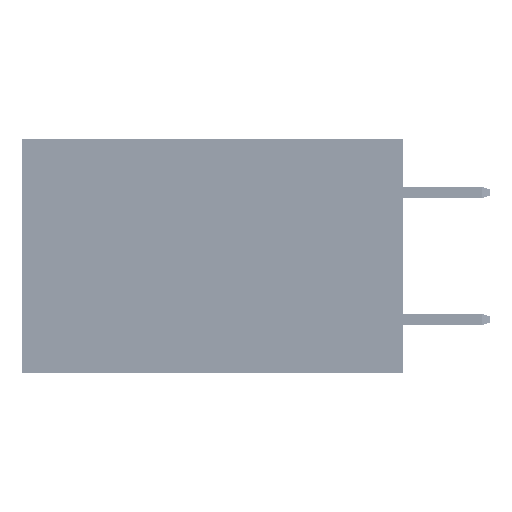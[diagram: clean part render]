
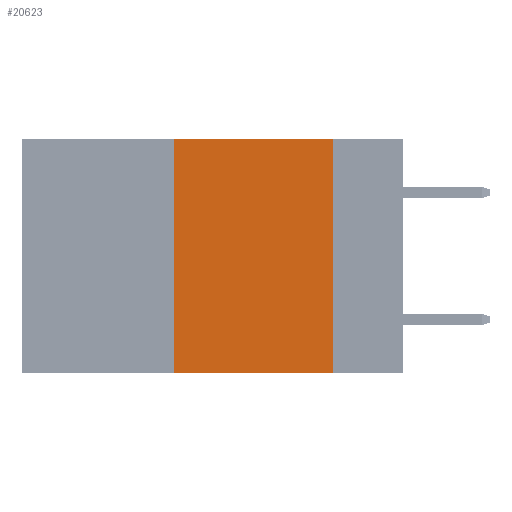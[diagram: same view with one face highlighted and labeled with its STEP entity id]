
A CAD part, left-side view. The second image highlights one B-rep face of the part: STEP entity #20623.
In plain terms, the highlighted planar face has unit normal (-1, 0, 0).
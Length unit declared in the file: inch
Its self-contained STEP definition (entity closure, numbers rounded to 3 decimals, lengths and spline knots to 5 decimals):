
#622 = CARTESIAN_POINT ( 'NONE',  ( 0., 0.6, 0. ) ) ;
#1249 = VECTOR ( 'NONE', #47459, 39.37008 ) ;
#1900 = DIRECTION ( 'NONE',  ( 0., -1., 0. ) ) ;
#4081 = ORIENTED_EDGE ( 'NONE', *, *, #17737, .T. ) ;
#5165 = VECTOR ( 'NONE', #27758, 39.37008 ) ;
#7792 = LINE ( 'NONE', #23218, #5165 ) ;
#12500 = DIRECTION ( 'NONE',  ( 1., 0., 0. ) ) ;
#12676 = AXIS2_PLACEMENT_3D ( 'NONE', #622, #12500, #43382 ) ;
#12749 = FACE_OUTER_BOUND ( 'NONE', #41569, .T. ) ;
#12773 = LINE ( 'NONE', #35773, #1249 ) ;
#14233 = CARTESIAN_POINT ( 'NONE',  ( 0., 0.6, -0.37 ) ) ;
#17259 = LINE ( 'NONE', #14233, #41562 ) ;
#17737 = EDGE_CURVE ( 'NONE', #49521, #19978, #17259, .T. ) ;
#19978 = VERTEX_POINT ( 'NONE', #49298 ) ;
#20623 = ADVANCED_FACE ( 'NONE', ( #12749 ), #46440, .F. ) ;
#21876 = ORIENTED_EDGE ( 'NONE', *, *, #36634, .F. ) ;
#23218 = CARTESIAN_POINT ( 'NONE',  ( 0., 0.36, 0. ) ) ;
#23468 = CARTESIAN_POINT ( 'NONE',  ( 0., 0.36, 0. ) ) ;
#23728 = CARTESIAN_POINT ( 'NONE',  ( 0., 0.11, 0. ) ) ;
#24161 = VERTEX_POINT ( 'NONE', #23728 ) ;
#25925 = CARTESIAN_POINT ( 'NONE',  ( 0., 0.6, 0. ) ) ;
#27758 = DIRECTION ( 'NONE',  ( 0., 0., 1. ) ) ;
#28663 = CARTESIAN_POINT ( 'NONE',  ( 0., 0.36, -0.37 ) ) ;
#30579 = ORIENTED_EDGE ( 'NONE', *, *, #47132, .F. ) ;
#33940 = VECTOR ( 'NONE', #1900, 39.37008 ) ;
#35773 = CARTESIAN_POINT ( 'NONE',  ( 0., 0.11, 0. ) ) ;
#36634 = EDGE_CURVE ( 'NONE', #49793, #24161, #48230, .T. ) ;
#37250 = DIRECTION ( 'NONE',  ( 0., -1., 0. ) ) ;
#41358 = ORIENTED_EDGE ( 'NONE', *, *, #49022, .F. ) ;
#41562 = VECTOR ( 'NONE', #37250, 39.37008 ) ;
#41569 = EDGE_LOOP ( 'NONE', ( #41358, #21876, #30579, #4081 ) ) ;
#43382 = DIRECTION ( 'NONE',  ( 0., 0., -1. ) ) ;
#46440 = PLANE ( 'NONE',  #12676 ) ;
#47132 = EDGE_CURVE ( 'NONE', #49521, #49793, #7792, .T. ) ;
#47459 = DIRECTION ( 'NONE',  ( 0., 0., -1. ) ) ;
#48230 = LINE ( 'NONE', #25925, #33940 ) ;
#49022 = EDGE_CURVE ( 'NONE', #24161, #19978, #12773, .T. ) ;
#49298 = CARTESIAN_POINT ( 'NONE',  ( 0., 0.11, -0.37 ) ) ;
#49521 = VERTEX_POINT ( 'NONE', #28663 ) ;
#49793 = VERTEX_POINT ( 'NONE', #23468 ) ;
